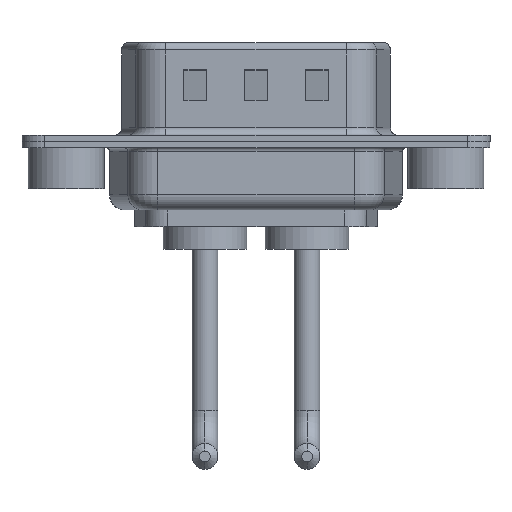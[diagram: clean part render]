
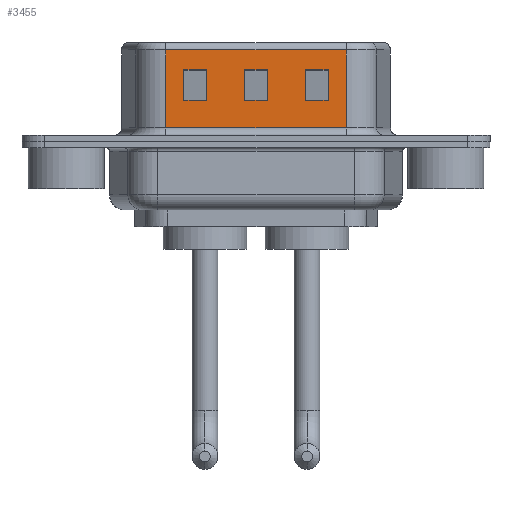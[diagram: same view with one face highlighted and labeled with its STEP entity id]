
A CAD part, front view. The second image highlights one B-rep face of the part: STEP entity #3455.
In plain terms, the highlighted planar face has unit normal (0, -1, 0).
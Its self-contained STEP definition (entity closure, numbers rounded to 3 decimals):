
#11 = EDGE_LOOP ( 'NONE', ( #9251, #11758, #13322, #4759 ) ) ;
#106 = LINE ( 'NONE', #6042, #12238 ) ;
#192 = LINE ( 'NONE', #1430, #4083 ) ;
#199 = DIRECTION ( 'NONE',  ( 0., 0., -1. ) ) ;
#317 = CARTESIAN_POINT ( 'NONE',  ( 6.549, -4.55, 6.02 ) ) ;
#323 = EDGE_CURVE ( 'NONE', #8350, #7971, #12526, .T. ) ;
#479 = CARTESIAN_POINT ( 'NONE',  ( 18.451, -4.55, 0.9 ) ) ;
#585 = FACE_OUTER_BOUND ( 'NONE', #14101, .T. ) ;
#589 = VECTOR ( 'NONE', #8207, 1000. ) ;
#664 = VERTEX_POINT ( 'NONE', #4917 ) ;
#682 = LINE ( 'NONE', #12838, #3383 ) ;
#712 = EDGE_CURVE ( 'NONE', #12464, #8707, #1465, .T. ) ;
#804 = CARTESIAN_POINT ( 'NONE',  ( 13.25, -4.55, 2.705 ) ) ;
#913 = DIRECTION ( 'NONE',  ( 0., 0., -1. ) ) ;
#1063 = VECTOR ( 'NONE', #199, 1000. ) ;
#1072 = VECTOR ( 'NONE', #11005, 1000. ) ;
#1177 = LINE ( 'NONE', #8996, #10371 ) ;
#1326 = LINE ( 'NONE', #4845, #5101 ) ;
#1430 = CARTESIAN_POINT ( 'NONE',  ( 18.451, -4.55, 0.9 ) ) ;
#1465 = LINE ( 'NONE', #2714, #589 ) ;
#1489 = DIRECTION ( 'NONE',  ( 0., 0., 1. ) ) ;
#1592 = EDGE_CURVE ( 'NONE', #12855, #11258, #1177, .T. ) ;
#1798 = EDGE_CURVE ( 'NONE', #6971, #13941, #682, .T. ) ;
#2026 = VECTOR ( 'NONE', #3037, 1000. ) ;
#2131 = VERTEX_POINT ( 'NONE', #10493 ) ;
#2270 = ORIENTED_EDGE ( 'NONE', *, *, #2391, .T. ) ;
#2391 = EDGE_CURVE ( 'NONE', #7971, #12855, #13173, .T. ) ;
#2452 = CARTESIAN_POINT ( 'NONE',  ( 17.25, -4.55, 4.705 ) ) ;
#2714 = CARTESIAN_POINT ( 'NONE',  ( 22.451, -4.55, 4.705 ) ) ;
#3037 = DIRECTION ( 'NONE',  ( 0., 0., 1. ) ) ;
#3312 = VECTOR ( 'NONE', #11934, 1000. ) ;
#3329 = CARTESIAN_POINT ( 'NONE',  ( 13.25, -4.55, 6.52 ) ) ;
#3383 = VECTOR ( 'NONE', #10883, 1000. ) ;
#3384 = EDGE_CURVE ( 'NONE', #2131, #9569, #9201, .T. ) ;
#3455 = ADVANCED_FACE ( 'NONE', ( #4831, #7317, #7251, #585 ), #5054, .F. ) ;
#3535 = CARTESIAN_POINT ( 'NONE',  ( 6.549, -4.55, 0.9 ) ) ;
#3978 = ORIENTED_EDGE ( 'NONE', *, *, #14053, .T. ) ;
#4083 = VECTOR ( 'NONE', #13456, 1000. ) ;
#4149 = CARTESIAN_POINT ( 'NONE',  ( 11.75, -4.55, 6.52 ) ) ;
#4226 = CARTESIAN_POINT ( 'NONE',  ( 7.75, -4.55, 4.705 ) ) ;
#4240 = CARTESIAN_POINT ( 'NONE',  ( 13.25, -4.55, 4.705 ) ) ;
#4246 = CARTESIAN_POINT ( 'NONE',  ( 15.75, -4.55, 4.705 ) ) ;
#4314 = VERTEX_POINT ( 'NONE', #479 ) ;
#4680 = CARTESIAN_POINT ( 'NONE',  ( 17.25, -4.55, 2.705 ) ) ;
#4689 = DIRECTION ( 'NONE',  ( -1., 0., 0. ) ) ;
#4759 = ORIENTED_EDGE ( 'NONE', *, *, #712, .T. ) ;
#4831 = FACE_BOUND ( 'NONE', #9784, .T. ) ;
#4845 = CARTESIAN_POINT ( 'NONE',  ( 18.451, -4.55, 6.52 ) ) ;
#4902 = DIRECTION ( 'NONE',  ( -1., 0., 0. ) ) ;
#4917 = CARTESIAN_POINT ( 'NONE',  ( 9.25, -4.55, 4.705 ) ) ;
#5054 = PLANE ( 'NONE',  #5571 ) ;
#5101 = VECTOR ( 'NONE', #9301, 1000. ) ;
#5364 = CARTESIAN_POINT ( 'NONE',  ( 9.25, -4.55, 2.705 ) ) ;
#5571 = AXIS2_PLACEMENT_3D ( 'NONE', #6002, #10436, #9287 ) ;
#5649 = ORIENTED_EDGE ( 'NONE', *, *, #1798, .T. ) ;
#5713 = EDGE_CURVE ( 'NONE', #8707, #9906, #10475, .T. ) ;
#6002 = CARTESIAN_POINT ( 'NONE',  ( 18.451, -4.55, 6.52 ) ) ;
#6012 = ORIENTED_EDGE ( 'NONE', *, *, #3384, .T. ) ;
#6042 = CARTESIAN_POINT ( 'NONE',  ( 15.75, -4.55, 6.52 ) ) ;
#6052 = VECTOR ( 'NONE', #4902, 1000. ) ;
#6216 = VECTOR ( 'NONE', #13158, 1000. ) ;
#6661 = VECTOR ( 'NONE', #11234, 1000. ) ;
#6896 = CARTESIAN_POINT ( 'NONE',  ( 11.75, -4.55, 2.705 ) ) ;
#6900 = VECTOR ( 'NONE', #14001, 1000. ) ;
#6971 = VERTEX_POINT ( 'NONE', #12920 ) ;
#7008 = CARTESIAN_POINT ( 'NONE',  ( 18.451, -4.55, 4.705 ) ) ;
#7096 = LINE ( 'NONE', #11526, #6900 ) ;
#7251 = FACE_BOUND ( 'NONE', #11806, .T. ) ;
#7269 = ORIENTED_EDGE ( 'NONE', *, *, #10542, .T. ) ;
#7317 = FACE_BOUND ( 'NONE', #11, .T. ) ;
#7782 = ORIENTED_EDGE ( 'NONE', *, *, #12692, .T. ) ;
#7826 = LINE ( 'NONE', #12257, #13645 ) ;
#7869 = LINE ( 'NONE', #14389, #6216 ) ;
#7971 = VERTEX_POINT ( 'NONE', #4240 ) ;
#8207 = DIRECTION ( 'NONE',  ( 1., 0., 0. ) ) ;
#8219 = EDGE_CURVE ( 'NONE', #9569, #11525, #12660, .T. ) ;
#8325 = CARTESIAN_POINT ( 'NONE',  ( 11.75, -4.55, 4.705 ) ) ;
#8350 = VERTEX_POINT ( 'NONE', #8325 ) ;
#8707 = VERTEX_POINT ( 'NONE', #2452 ) ;
#8737 = LINE ( 'NONE', #4149, #2026 ) ;
#8996 = CARTESIAN_POINT ( 'NONE',  ( 18.451, -4.55, 2.705 ) ) ;
#9060 = CARTESIAN_POINT ( 'NONE',  ( 14.451, -4.55, 2.705 ) ) ;
#9120 = EDGE_CURVE ( 'NONE', #11027, #12464, #106, .T. ) ;
#9201 = LINE ( 'NONE', #12608, #6052 ) ;
#9251 = ORIENTED_EDGE ( 'NONE', *, *, #5713, .T. ) ;
#9287 = DIRECTION ( 'NONE',  ( -1., 0., 0. ) ) ;
#9301 = DIRECTION ( 'NONE',  ( 0., 0., -1. ) ) ;
#9526 = EDGE_CURVE ( 'NONE', #9906, #11027, #7869, .T. ) ;
#9569 = VERTEX_POINT ( 'NONE', #317 ) ;
#9764 = ORIENTED_EDGE ( 'NONE', *, *, #12131, .F. ) ;
#9784 = EDGE_LOOP ( 'NONE', ( #10816, #10044, #5649, #7782 ) ) ;
#9906 = VERTEX_POINT ( 'NONE', #4680 ) ;
#9988 = EDGE_CURVE ( 'NONE', #664, #11874, #7826, .T. ) ;
#10044 = ORIENTED_EDGE ( 'NONE', *, *, #12638, .T. ) ;
#10122 = CARTESIAN_POINT ( 'NONE',  ( 6.549, -4.55, 6.52 ) ) ;
#10371 = VECTOR ( 'NONE', #4689, 1000. ) ;
#10436 = DIRECTION ( 'NONE',  ( 0., 1., 0. ) ) ;
#10475 = LINE ( 'NONE', #13903, #3312 ) ;
#10493 = CARTESIAN_POINT ( 'NONE',  ( 18.451, -4.55, 6.02 ) ) ;
#10542 = EDGE_CURVE ( 'NONE', #11258, #8350, #8737, .T. ) ;
#10745 = ORIENTED_EDGE ( 'NONE', *, *, #1592, .T. ) ;
#10797 = VECTOR ( 'NONE', #12876, 1000. ) ;
#10816 = ORIENTED_EDGE ( 'NONE', *, *, #9988, .T. ) ;
#10883 = DIRECTION ( 'NONE',  ( 0., 0., 1. ) ) ;
#11005 = DIRECTION ( 'NONE',  ( 0., 0., -1. ) ) ;
#11027 = VERTEX_POINT ( 'NONE', #13073 ) ;
#11234 = DIRECTION ( 'NONE',  ( -1., 0., 0. ) ) ;
#11258 = VERTEX_POINT ( 'NONE', #6896 ) ;
#11525 = VERTEX_POINT ( 'NONE', #3535 ) ;
#11526 = CARTESIAN_POINT ( 'NONE',  ( 14.451, -4.55, 4.705 ) ) ;
#11758 = ORIENTED_EDGE ( 'NONE', *, *, #9526, .T. ) ;
#11806 = EDGE_LOOP ( 'NONE', ( #13085, #2270, #10745, #7269 ) ) ;
#11874 = VERTEX_POINT ( 'NONE', #5364 ) ;
#11934 = DIRECTION ( 'NONE',  ( 0., 0., -1. ) ) ;
#12131 = EDGE_CURVE ( 'NONE', #2131, #4314, #1326, .T. ) ;
#12238 = VECTOR ( 'NONE', #1489, 1000. ) ;
#12257 = CARTESIAN_POINT ( 'NONE',  ( 9.25, -4.55, 6.52 ) ) ;
#12464 = VERTEX_POINT ( 'NONE', #4246 ) ;
#12465 = LINE ( 'NONE', #9060, #6661 ) ;
#12526 = LINE ( 'NONE', #7008, #10797 ) ;
#12608 = CARTESIAN_POINT ( 'NONE',  ( 18.451, -4.55, 6.02 ) ) ;
#12638 = EDGE_CURVE ( 'NONE', #11874, #6971, #12465, .T. ) ;
#12660 = LINE ( 'NONE', #10122, #1063 ) ;
#12692 = EDGE_CURVE ( 'NONE', #13941, #664, #7096, .T. ) ;
#12838 = CARTESIAN_POINT ( 'NONE',  ( 7.75, -4.55, 6.52 ) ) ;
#12855 = VERTEX_POINT ( 'NONE', #804 ) ;
#12876 = DIRECTION ( 'NONE',  ( 1., 0., 0. ) ) ;
#12920 = CARTESIAN_POINT ( 'NONE',  ( 7.75, -4.55, 2.705 ) ) ;
#13073 = CARTESIAN_POINT ( 'NONE',  ( 15.75, -4.55, 2.705 ) ) ;
#13085 = ORIENTED_EDGE ( 'NONE', *, *, #323, .T. ) ;
#13158 = DIRECTION ( 'NONE',  ( -1., 0., 0. ) ) ;
#13173 = LINE ( 'NONE', #3329, #1072 ) ;
#13322 = ORIENTED_EDGE ( 'NONE', *, *, #9120, .T. ) ;
#13456 = DIRECTION ( 'NONE',  ( 1., 0., 0. ) ) ;
#13645 = VECTOR ( 'NONE', #913, 1000. ) ;
#13903 = CARTESIAN_POINT ( 'NONE',  ( 17.25, -4.55, 6.52 ) ) ;
#13941 = VERTEX_POINT ( 'NONE', #4226 ) ;
#13946 = ORIENTED_EDGE ( 'NONE', *, *, #8219, .T. ) ;
#14001 = DIRECTION ( 'NONE',  ( 1., 0., 0. ) ) ;
#14053 = EDGE_CURVE ( 'NONE', #11525, #4314, #192, .T. ) ;
#14101 = EDGE_LOOP ( 'NONE', ( #9764, #6012, #13946, #3978 ) ) ;
#14389 = CARTESIAN_POINT ( 'NONE',  ( 22.451, -4.55, 2.705 ) ) ;
